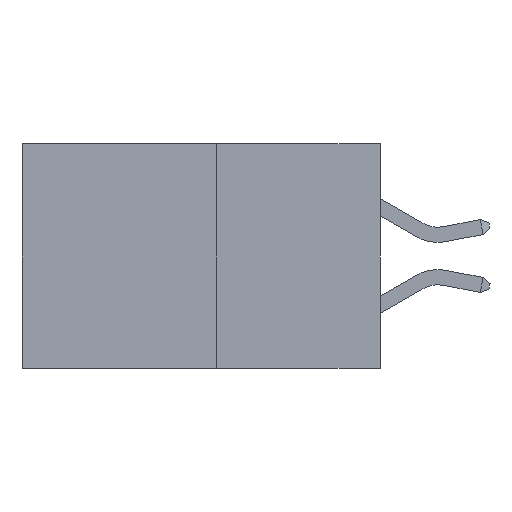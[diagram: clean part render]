
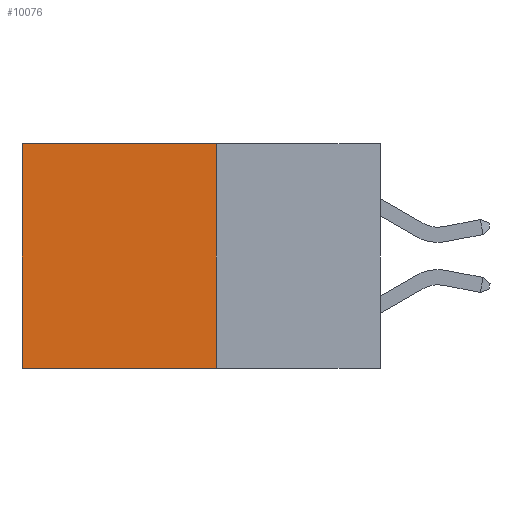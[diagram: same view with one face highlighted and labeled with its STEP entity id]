
A CAD part, left-side view. The second image highlights one B-rep face of the part: STEP entity #10076.
In plain terms, the highlighted planar face has unit normal (-1, 0, 0).
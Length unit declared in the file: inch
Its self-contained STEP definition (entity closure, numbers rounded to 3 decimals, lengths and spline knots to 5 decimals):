
#718 = CARTESIAN_POINT ( 'NONE',  ( 0.277, 0.27, -0.37 ) ) ;
#730 = EDGE_CURVE ( 'NONE', #23693, #6060, #1373, .T. ) ;
#1373 = LINE ( 'NONE', #22951, #22787 ) ;
#2071 = VECTOR ( 'NONE', #8242, 39.37008 ) ;
#2858 = PLANE ( 'NONE',  #7727 ) ;
#2910 = CARTESIAN_POINT ( 'NONE',  ( 0.277, 0.27, -0.37 ) ) ;
#2976 = DIRECTION ( 'NONE',  ( 1., 0., 0. ) ) ;
#3015 = DIRECTION ( 'NONE',  ( 0., 0., -1. ) ) ;
#6060 = VERTEX_POINT ( 'NONE', #20727 ) ;
#6238 = VECTOR ( 'NONE', #6644, 39.37008 ) ;
#6644 = DIRECTION ( 'NONE',  ( 0., 0., -1. ) ) ;
#7154 = CARTESIAN_POINT ( 'NONE',  ( 0.277, 0.59, -0.37 ) ) ;
#7560 = EDGE_CURVE ( 'NONE', #11448, #23693, #19791, .T. ) ;
#7644 = EDGE_CURVE ( 'NONE', #16050, #6060, #22598, .T. ) ;
#7723 = ORIENTED_EDGE ( 'NONE', *, *, #9683, .T. ) ;
#7727 = AXIS2_PLACEMENT_3D ( 'NONE', #2910, #2976, #3015 ) ;
#8087 = FACE_OUTER_BOUND ( 'NONE', #13512, .T. ) ;
#8242 = DIRECTION ( 'NONE',  ( 0., 1., 0. ) ) ;
#8272 = CARTESIAN_POINT ( 'NONE',  ( 0.277, 0.27, 0. ) ) ;
#9136 = DIRECTION ( 'NONE',  ( 0., 0., -1. ) ) ;
#9262 = CARTESIAN_POINT ( 'NONE',  ( 0.277, 0.27, -0.37 ) ) ;
#9683 = EDGE_CURVE ( 'NONE', #11448, #16050, #23476, .T. ) ;
#10076 = ADVANCED_FACE ( 'NONE', ( #8087 ), #2858, .F. ) ;
#11448 = VERTEX_POINT ( 'NONE', #19649 ) ;
#13512 = EDGE_LOOP ( 'NONE', ( #24829, #18307, #18821, #7723 ) ) ;
#16050 = VERTEX_POINT ( 'NONE', #18366 ) ;
#18307 = ORIENTED_EDGE ( 'NONE', *, *, #730, .F. ) ;
#18366 = CARTESIAN_POINT ( 'NONE',  ( 0.277, 0.59, 0. ) ) ;
#18821 = ORIENTED_EDGE ( 'NONE', *, *, #7560, .F. ) ;
#19178 = VECTOR ( 'NONE', #9136, 39.37008 ) ;
#19649 = CARTESIAN_POINT ( 'NONE',  ( 0.277, 0.27, 0. ) ) ;
#19791 = LINE ( 'NONE', #9262, #19178 ) ;
#20727 = CARTESIAN_POINT ( 'NONE',  ( 0.277, 0.59, -0.37 ) ) ;
#22222 = DIRECTION ( 'NONE',  ( 0., 1., 0. ) ) ;
#22598 = LINE ( 'NONE', #7154, #6238 ) ;
#22787 = VECTOR ( 'NONE', #22222, 39.37008 ) ;
#22951 = CARTESIAN_POINT ( 'NONE',  ( 0.277, 0.27, -0.37 ) ) ;
#23476 = LINE ( 'NONE', #8272, #2071 ) ;
#23693 = VERTEX_POINT ( 'NONE', #718 ) ;
#24829 = ORIENTED_EDGE ( 'NONE', *, *, #7644, .T. ) ;
